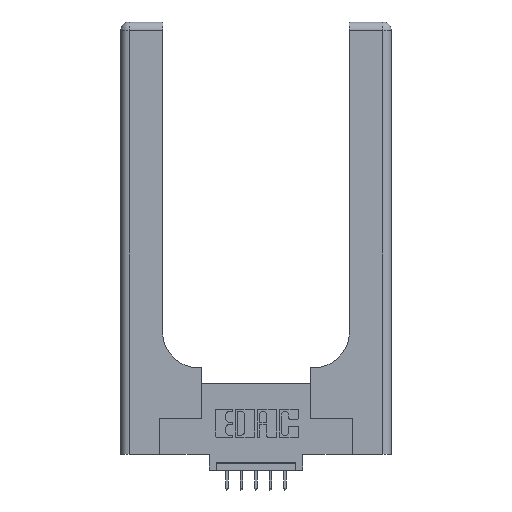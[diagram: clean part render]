
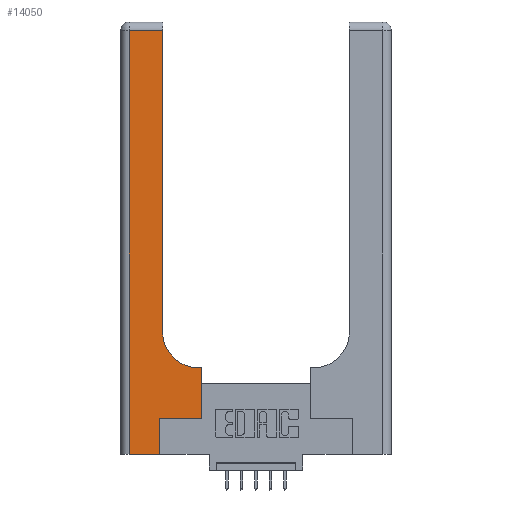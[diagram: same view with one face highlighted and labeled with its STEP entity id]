
A CAD part, top view. The second image highlights one B-rep face of the part: STEP entity #14050.
In plain terms, the highlighted planar face has unit normal (0, 0, 1).
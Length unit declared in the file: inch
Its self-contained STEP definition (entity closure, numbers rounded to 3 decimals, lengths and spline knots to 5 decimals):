
#137 = CARTESIAN_POINT ( 'NONE',  ( 0.5585, 0.6, 0.37 ) ) ;
#196 = CARTESIAN_POINT ( 'NONE',  ( 0.269, 0.25, 0.37 ) ) ;
#994 = CARTESIAN_POINT ( 'NONE',  ( 0.5415, 0.85, 0.37 ) ) ;
#1046 = LINE ( 'NONE', #4316, #4109 ) ;
#1056 = LINE ( 'NONE', #6323, #4891 ) ;
#1086 = VERTEX_POINT ( 'NONE', #4285 ) ;
#1184 = ORIENTED_EDGE ( 'NONE', *, *, #11778, .T. ) ;
#1254 = DIRECTION ( 'NONE',  ( -1., 0., 0. ) ) ;
#1494 = VERTEX_POINT ( 'NONE', #137 ) ;
#1942 = VERTEX_POINT ( 'NONE', #5066 ) ;
#1983 = DIRECTION ( 'NONE',  ( 0., 1., 0. ) ) ;
#2047 = LINE ( 'NONE', #6402, #13050 ) ;
#2080 = CIRCLE ( 'NONE', #8279, 0.25 ) ;
#2115 = DIRECTION ( 'NONE',  ( 0., -1., 0. ) ) ;
#2172 = CARTESIAN_POINT ( 'NONE',  ( 0.269, 0., 0.37 ) ) ;
#2607 = ORIENTED_EDGE ( 'NONE', *, *, #9532, .T. ) ;
#2626 = LINE ( 'NONE', #4828, #7109 ) ;
#2675 = LINE ( 'NONE', #4602, #4342 ) ;
#3425 = DIRECTION ( 'NONE',  ( 1., 0., 0. ) ) ;
#3753 = VERTEX_POINT ( 'NONE', #4029 ) ;
#3758 = VECTOR ( 'NONE', #8499, 39.37008 ) ;
#4029 = CARTESIAN_POINT ( 'NONE',  ( 0.2915, 0.85, 0.37 ) ) ;
#4109 = VECTOR ( 'NONE', #8710, 39.37008 ) ;
#4285 = CARTESIAN_POINT ( 'NONE',  ( 0.269, 0.25, 0.37 ) ) ;
#4316 = CARTESIAN_POINT ( 'NONE',  ( 0.2915, 3., 0.37 ) ) ;
#4342 = VECTOR ( 'NONE', #1254, 39.37008 ) ;
#4439 = DIRECTION ( 'NONE',  ( 0., 0., -1. ) ) ;
#4512 = VERTEX_POINT ( 'NONE', #8008 ) ;
#4602 = CARTESIAN_POINT ( 'NONE',  ( 0., 2.94, 0.37 ) ) ;
#4628 = ORIENTED_EDGE ( 'NONE', *, *, #13598, .T. ) ;
#4828 = CARTESIAN_POINT ( 'NONE',  ( 0.5585, 0.25, 0.37 ) ) ;
#4891 = VECTOR ( 'NONE', #2115, 39.37008 ) ;
#5066 = CARTESIAN_POINT ( 'NONE',  ( 0.5585, 0.25, 0.37 ) ) ;
#5126 = EDGE_LOOP ( 'NONE', ( #6448, #2607, #11802, #4628, #7344, #5145, #11262, #1184, #11023 ) ) ;
#5145 = ORIENTED_EDGE ( 'NONE', *, *, #11170, .T. ) ;
#5815 = AXIS2_PLACEMENT_3D ( 'NONE', #11962, #4439, #9979 ) ;
#6088 = EDGE_CURVE ( 'NONE', #11877, #1086, #2047, .T. ) ;
#6100 = EDGE_CURVE ( 'NONE', #6620, #3753, #2080, .T. ) ;
#6227 = EDGE_CURVE ( 'NONE', #1942, #1494, #2626, .T. ) ;
#6308 = CARTESIAN_POINT ( 'NONE',  ( 0.2915, 0.6, 0.37 ) ) ;
#6323 = CARTESIAN_POINT ( 'NONE',  ( 0.06, 3., 0.37 ) ) ;
#6402 = CARTESIAN_POINT ( 'NONE',  ( 0.269, 0., 0.37 ) ) ;
#6448 = ORIENTED_EDGE ( 'NONE', *, *, #7379, .T. ) ;
#6596 = LINE ( 'NONE', #6308, #7848 ) ;
#6620 = VERTEX_POINT ( 'NONE', #9833 ) ;
#7109 = VECTOR ( 'NONE', #9223, 39.37008 ) ;
#7156 = CARTESIAN_POINT ( 'NONE',  ( 0.06, 2.94, 0.37 ) ) ;
#7344 = ORIENTED_EDGE ( 'NONE', *, *, #6088, .T. ) ;
#7379 = EDGE_CURVE ( 'NONE', #3753, #4512, #1046, .T. ) ;
#7670 = PLANE ( 'NONE',  #5815 ) ;
#7848 = VECTOR ( 'NONE', #12057, 39.37008 ) ;
#8008 = CARTESIAN_POINT ( 'NONE',  ( 0.2915, 2.94, 0.37 ) ) ;
#8279 = AXIS2_PLACEMENT_3D ( 'NONE', #994, #9743, #11942 ) ;
#8499 = DIRECTION ( 'NONE',  ( 1., 0., 0. ) ) ;
#8710 = DIRECTION ( 'NONE',  ( 0., 1., 0. ) ) ;
#9223 = DIRECTION ( 'NONE',  ( 0., 1., 0. ) ) ;
#9532 = EDGE_CURVE ( 'NONE', #4512, #12326, #2675, .T. ) ;
#9743 = DIRECTION ( 'NONE',  ( 0., 0., -1. ) ) ;
#9826 = CARTESIAN_POINT ( 'NONE',  ( 0.06, 0., 0.37 ) ) ;
#9833 = CARTESIAN_POINT ( 'NONE',  ( 0.5415, 0.6, 0.37 ) ) ;
#9942 = CARTESIAN_POINT ( 'NONE',  ( 0., 0., 0.37 ) ) ;
#9979 = DIRECTION ( 'NONE',  ( -1., 0., 0. ) ) ;
#11023 = ORIENTED_EDGE ( 'NONE', *, *, #6100, .T. ) ;
#11030 = LINE ( 'NONE', #196, #11503 ) ;
#11170 = EDGE_CURVE ( 'NONE', #1086, #1942, #11030, .T. ) ;
#11262 = ORIENTED_EDGE ( 'NONE', *, *, #6227, .T. ) ;
#11503 = VECTOR ( 'NONE', #3425, 39.37008 ) ;
#11778 = EDGE_CURVE ( 'NONE', #1494, #6620, #6596, .T. ) ;
#11788 = LINE ( 'NONE', #9942, #3758 ) ;
#11802 = ORIENTED_EDGE ( 'NONE', *, *, #13609, .T. ) ;
#11877 = VERTEX_POINT ( 'NONE', #2172 ) ;
#11942 = DIRECTION ( 'NONE',  ( 1., 0., 0. ) ) ;
#11962 = CARTESIAN_POINT ( 'NONE',  ( 0., 3., 0.37 ) ) ;
#12057 = DIRECTION ( 'NONE',  ( -1., 0., 0. ) ) ;
#12326 = VERTEX_POINT ( 'NONE', #7156 ) ;
#13050 = VECTOR ( 'NONE', #1983, 39.37008 ) ;
#13100 = FACE_OUTER_BOUND ( 'NONE', #5126, .T. ) ;
#13598 = EDGE_CURVE ( 'NONE', #14108, #11877, #11788, .T. ) ;
#13609 = EDGE_CURVE ( 'NONE', #12326, #14108, #1056, .T. ) ;
#14050 = ADVANCED_FACE ( 'NONE', ( #13100 ), #7670, .F. ) ;
#14108 = VERTEX_POINT ( 'NONE', #9826 ) ;
